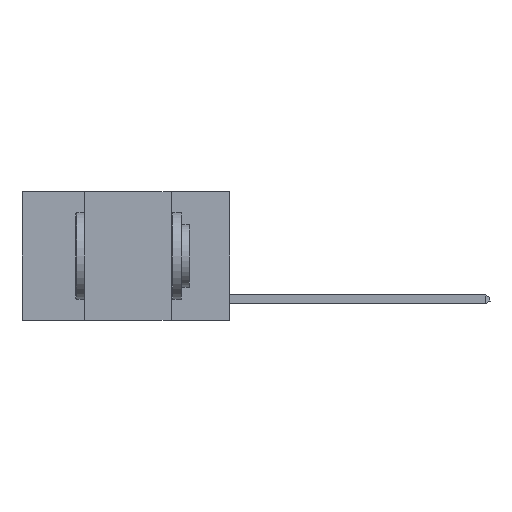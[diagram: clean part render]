
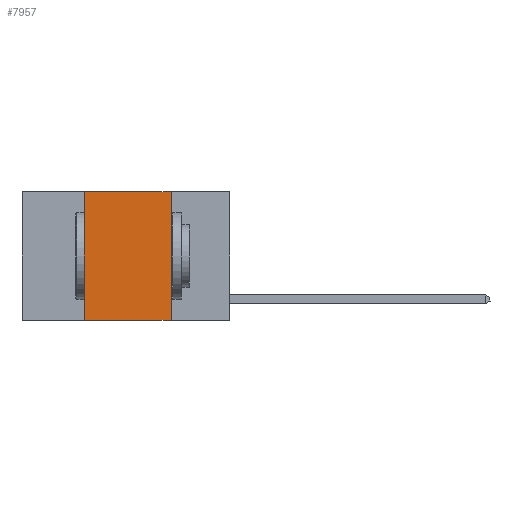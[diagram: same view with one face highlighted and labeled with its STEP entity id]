
A CAD part, left-side view. The second image highlights one B-rep face of the part: STEP entity #7957.
In plain terms, the highlighted planar face has unit normal (-1, 0, 0).
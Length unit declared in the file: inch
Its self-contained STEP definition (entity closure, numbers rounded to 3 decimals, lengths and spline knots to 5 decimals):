
#408 = VERTEX_POINT ( 'NONE', #2831 ) ;
#1166 = DIRECTION ( 'NONE',  ( 1., 0., 0. ) ) ;
#1216 = FACE_OUTER_BOUND ( 'NONE', #6729, .T. ) ;
#1655 = ORIENTED_EDGE ( 'NONE', *, *, #6272, .F. ) ;
#2294 = VECTOR ( 'NONE', #3373, 39.37008 ) ;
#2544 = CARTESIAN_POINT ( 'NONE',  ( 0., 0.6, -0.37 ) ) ;
#2831 = CARTESIAN_POINT ( 'NONE',  ( 0., 0.42, 0. ) ) ;
#2869 = CARTESIAN_POINT ( 'NONE',  ( 0., 0.42, -0.37 ) ) ;
#2912 = VECTOR ( 'NONE', #3291, 39.37008 ) ;
#3114 = AXIS2_PLACEMENT_3D ( 'NONE', #7932, #1166, #4159 ) ;
#3291 = DIRECTION ( 'NONE',  ( 0., 0., 1. ) ) ;
#3373 = DIRECTION ( 'NONE',  ( 0., -1., 0. ) ) ;
#4130 = LINE ( 'NONE', #2544, #2294 ) ;
#4159 = DIRECTION ( 'NONE',  ( 0., 0., -1. ) ) ;
#4562 = EDGE_CURVE ( 'NONE', #5648, #5547, #5508, .T. ) ;
#4994 = VERTEX_POINT ( 'NONE', #2869 ) ;
#5330 = CARTESIAN_POINT ( 'NONE',  ( 0., 0.6, 0. ) ) ;
#5508 = LINE ( 'NONE', #6192, #8753 ) ;
#5547 = VERTEX_POINT ( 'NONE', #9594 ) ;
#5648 = VERTEX_POINT ( 'NONE', #9095 ) ;
#6022 = ORIENTED_EDGE ( 'NONE', *, *, #8736, .T. ) ;
#6192 = CARTESIAN_POINT ( 'NONE',  ( 0., 0.17, 0. ) ) ;
#6248 = DIRECTION ( 'NONE',  ( 0., 0., -1. ) ) ;
#6272 = EDGE_CURVE ( 'NONE', #4994, #408, #7718, .T. ) ;
#6612 = ORIENTED_EDGE ( 'NONE', *, *, #8788, .F. ) ;
#6729 = EDGE_LOOP ( 'NONE', ( #8352, #6612, #1655, #6022 ) ) ;
#7030 = CARTESIAN_POINT ( 'NONE',  ( 0., 0.42, 0. ) ) ;
#7247 = PLANE ( 'NONE',  #3114 ) ;
#7599 = LINE ( 'NONE', #5330, #7959 ) ;
#7718 = LINE ( 'NONE', #7030, #2912 ) ;
#7932 = CARTESIAN_POINT ( 'NONE',  ( 0., 0.6, 0. ) ) ;
#7957 = ADVANCED_FACE ( 'NONE', ( #1216 ), #7247, .F. ) ;
#7959 = VECTOR ( 'NONE', #8018, 39.37008 ) ;
#8018 = DIRECTION ( 'NONE',  ( 0., -1., 0. ) ) ;
#8352 = ORIENTED_EDGE ( 'NONE', *, *, #4562, .F. ) ;
#8736 = EDGE_CURVE ( 'NONE', #4994, #5547, #4130, .T. ) ;
#8753 = VECTOR ( 'NONE', #6248, 39.37008 ) ;
#8788 = EDGE_CURVE ( 'NONE', #408, #5648, #7599, .T. ) ;
#9095 = CARTESIAN_POINT ( 'NONE',  ( 0., 0.17, 0. ) ) ;
#9594 = CARTESIAN_POINT ( 'NONE',  ( 0., 0.17, -0.37 ) ) ;
